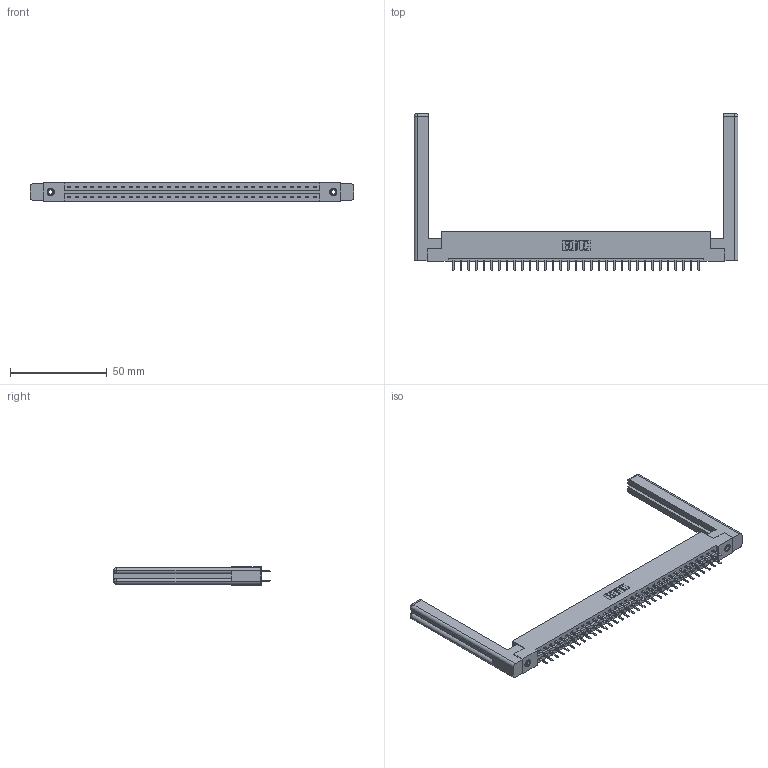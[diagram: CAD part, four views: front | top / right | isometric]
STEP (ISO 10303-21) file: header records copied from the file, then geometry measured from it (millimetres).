
FILE_DESCRIPTION (( 'STEP AP203' ), '1' );
FILE_NAME ('387-066-520-258.STEP', '2019-10-19T17:58:56', ( '' ), ( '' ), 'SwSTEP 2.0', 'SolidWorks 2016', '' );
FILE_SCHEMA (( 'CONFIG_CONTROL_DESIGN' ));
Length unit declared in the file: inch
Products named in the file (5): 345-250-001_345-250-001-102; 307-220-058; 387-066-520-258; 345-292-001_345-293-120; 337 Part_Flush Mounting Lugs - 0.156 Dia-TI
Assembly tree (71 placements, depth 2):
  387-066-520-258
    337 Part_Flush Mounting Lugs - 0.156 Dia-TI
    345-292-001_345-293-120  x66
    345-250-001_345-250-001-102  x2
    307-220-058  x2
Bounding box: 167.39 x 81.11 x 9.4 mm (x, y, z)
Volume: 24634 mm3; surface area: 24650.9 mm2
Topology: 71 solids, 71 shells, 4084 faces, 11819 edges, 7690 vertices
Faces by surface type: plane 2794, cylinder 1266, cone 12, torus 12
Entity records: 29498 total; most frequent: CARTESIAN_POINT 4997, ORIENTED_EDGE 4860, DIRECTION 4270, EDGE_CURVE 2430, LINE 2250, VECTOR 2250, VERTEX_POINT 1610, AXIS2_PLACEMENT_3D 1010
